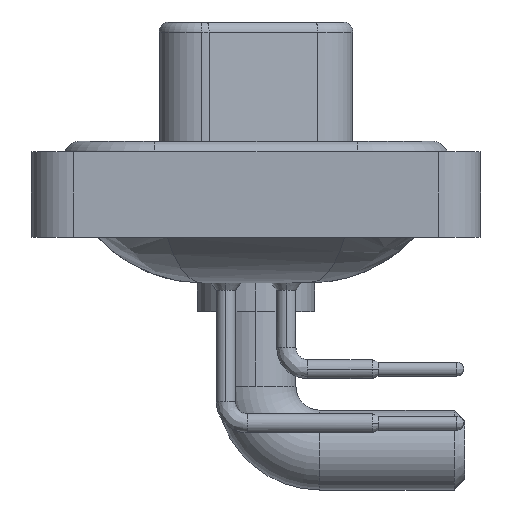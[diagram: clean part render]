
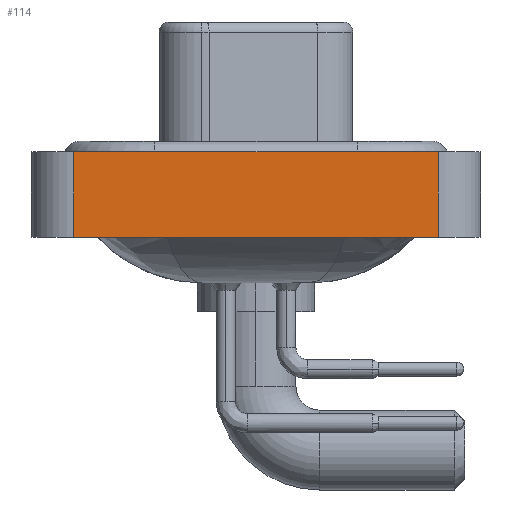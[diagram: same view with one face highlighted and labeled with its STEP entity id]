
A CAD part, left-side view. The second image highlights one B-rep face of the part: STEP entity #114.
In plain terms, the highlighted planar face has unit normal (-1, 0, 0).
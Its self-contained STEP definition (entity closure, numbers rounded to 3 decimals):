
#114 = ADVANCED_FACE ( 'NONE', ( #8269 ), #28897, .T. ) ;
#1854 = VERTEX_POINT ( 'NONE', #24487 ) ;
#2514 = AXIS2_PLACEMENT_3D ( 'NONE', #3785, #10932, #17491 ) ;
#2556 = CARTESIAN_POINT ( 'NONE',  ( -7.35, -8.55, -3.6 ) ) ;
#3614 = EDGE_LOOP ( 'NONE', ( #19100, #16080, #12508, #19430 ) ) ;
#3785 = CARTESIAN_POINT ( 'NONE',  ( -7.35, -8.55, -3.6 ) ) ;
#4024 = VECTOR ( 'NONE', #5411, 1000. ) ;
#5411 = DIRECTION ( 'NONE',  ( 0., 0., 1. ) ) ;
#7504 = CARTESIAN_POINT ( 'NONE',  ( -7.35, 8.55, -3.6 ) ) ;
#7795 = LINE ( 'NONE', #24064, #23321 ) ;
#7829 = VERTEX_POINT ( 'NONE', #16569 ) ;
#7949 = DIRECTION ( 'NONE',  ( 0., 0., 1. ) ) ;
#8269 = FACE_OUTER_BOUND ( 'NONE', #3614, .T. ) ;
#8835 = DIRECTION ( 'NONE',  ( 0., -1., 0. ) ) ;
#9606 = VERTEX_POINT ( 'NONE', #12351 ) ;
#9869 = DIRECTION ( 'NONE',  ( 0., -1., 0. ) ) ;
#10932 = DIRECTION ( 'NONE',  ( -1., 0., 0. ) ) ;
#11303 = CARTESIAN_POINT ( 'NONE',  ( -7.35, 8.55, -3.6 ) ) ;
#11889 = VECTOR ( 'NONE', #8835, 1000. ) ;
#12351 = CARTESIAN_POINT ( 'NONE',  ( -7.35, 8.55, 0.4 ) ) ;
#12508 = ORIENTED_EDGE ( 'NONE', *, *, #17354, .F. ) ;
#14638 = VECTOR ( 'NONE', #9869, 1000. ) ;
#16080 = ORIENTED_EDGE ( 'NONE', *, *, #19706, .F. ) ;
#16569 = CARTESIAN_POINT ( 'NONE',  ( -7.35, -8.55, 0.4 ) ) ;
#17354 = EDGE_CURVE ( 'NONE', #26727, #9606, #27577, .T. ) ;
#17491 = DIRECTION ( 'NONE',  ( 0., 0., 1. ) ) ;
#19100 = ORIENTED_EDGE ( 'NONE', *, *, #19538, .T. ) ;
#19430 = ORIENTED_EDGE ( 'NONE', *, *, #24660, .T. ) ;
#19538 = EDGE_CURVE ( 'NONE', #1854, #7829, #7795, .T. ) ;
#19706 = EDGE_CURVE ( 'NONE', #9606, #7829, #20317, .T. ) ;
#20317 = LINE ( 'NONE', #29469, #11889 ) ;
#22862 = LINE ( 'NONE', #2556, #14638 ) ;
#23321 = VECTOR ( 'NONE', #7949, 1000. ) ;
#24064 = CARTESIAN_POINT ( 'NONE',  ( -7.35, -8.55, -3.6 ) ) ;
#24487 = CARTESIAN_POINT ( 'NONE',  ( -7.35, -8.55, -3.6 ) ) ;
#24660 = EDGE_CURVE ( 'NONE', #26727, #1854, #22862, .T. ) ;
#26727 = VERTEX_POINT ( 'NONE', #11303 ) ;
#27577 = LINE ( 'NONE', #7504, #4024 ) ;
#28897 = PLANE ( 'NONE',  #2514 ) ;
#29469 = CARTESIAN_POINT ( 'NONE',  ( -7.35, -8.55, 0.4 ) ) ;
